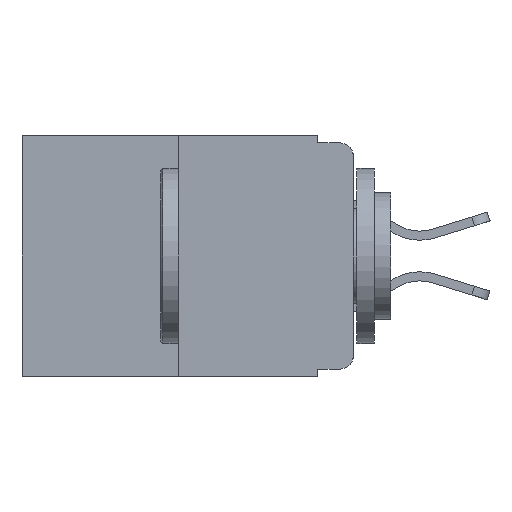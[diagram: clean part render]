
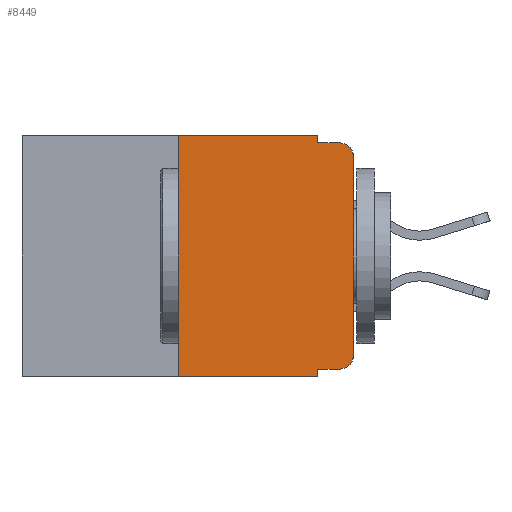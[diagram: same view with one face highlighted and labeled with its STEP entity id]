
A CAD part, left-side view. The second image highlights one B-rep face of the part: STEP entity #8449.
In plain terms, the highlighted planar face has unit normal (-1, 0, 0).
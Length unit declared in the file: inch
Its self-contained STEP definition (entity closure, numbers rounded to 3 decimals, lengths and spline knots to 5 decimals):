
#26 = CARTESIAN_POINT ( 'NONE',  ( 0., 0., -0.313 ) ) ;
#268 = ORIENTED_EDGE ( 'NONE', *, *, #11243, .T. ) ;
#380 = EDGE_CURVE ( 'NONE', #701, #8405, #5730, .T. ) ;
#486 = DIRECTION ( 'NONE',  ( 0., -1., 0. ) ) ;
#609 = CARTESIAN_POINT ( 'NONE',  ( 0., 0.051, -0.01 ) ) ;
#701 = VERTEX_POINT ( 'NONE', #7316 ) ;
#868 = LINE ( 'NONE', #9884, #1958 ) ;
#952 = CARTESIAN_POINT ( 'NONE',  ( 0., 0., -0.03 ) ) ;
#1090 = ORIENTED_EDGE ( 'NONE', *, *, #380, .F. ) ;
#1113 = DIRECTION ( 'NONE',  ( 0., 0., 1. ) ) ;
#1114 = CARTESIAN_POINT ( 'NONE',  ( 0., 0.051, 0. ) ) ;
#1180 = EDGE_CURVE ( 'NONE', #1387, #6150, #7478, .T. ) ;
#1249 = VERTEX_POINT ( 'NONE', #9430 ) ;
#1387 = VERTEX_POINT ( 'NONE', #9670 ) ;
#1479 = EDGE_LOOP ( 'NONE', ( #268, #3017, #3882, #7812, #5936, #1090, #8109, #7194, #1755, #11623 ) ) ;
#1579 = VERTEX_POINT ( 'NONE', #1114 ) ;
#1755 = ORIENTED_EDGE ( 'NONE', *, *, #5797, .T. ) ;
#1958 = VECTOR ( 'NONE', #5433, 39.37008 ) ;
#2484 = CARTESIAN_POINT ( 'NONE',  ( 0., 0.02, -0.333 ) ) ;
#2548 = LINE ( 'NONE', #6220, #4868 ) ;
#2768 = VECTOR ( 'NONE', #3510, 39.37008 ) ;
#2850 = LINE ( 'NONE', #7996, #2768 ) ;
#2852 = FACE_OUTER_BOUND ( 'NONE', #1479, .T. ) ;
#2918 = CIRCLE ( 'NONE', #11065, 0.02 ) ;
#3017 = ORIENTED_EDGE ( 'NONE', *, *, #8874, .T. ) ;
#3197 = VECTOR ( 'NONE', #4030, 39.37008 ) ;
#3454 = CARTESIAN_POINT ( 'NONE',  ( 0., 0.02, -0.313 ) ) ;
#3510 = DIRECTION ( 'NONE',  ( 0., -1., 0. ) ) ;
#3515 = EDGE_CURVE ( 'NONE', #8405, #1579, #10163, .T. ) ;
#3670 = DIRECTION ( 'NONE',  ( 0., 0., -1. ) ) ;
#3882 = ORIENTED_EDGE ( 'NONE', *, *, #10359, .F. ) ;
#3915 = DIRECTION ( 'NONE',  ( 0., 0., -1. ) ) ;
#4030 = DIRECTION ( 'NONE',  ( 0., 0., -1. ) ) ;
#4073 = EDGE_CURVE ( 'NONE', #701, #6150, #2850, .T. ) ;
#4125 = CARTESIAN_POINT ( 'NONE',  ( 0., 0.051, -0.343 ) ) ;
#4605 = CIRCLE ( 'NONE', #6100, 0.02 ) ;
#4614 = CARTESIAN_POINT ( 'NONE',  ( 0., 0.02, -0.03 ) ) ;
#4632 = AXIS2_PLACEMENT_3D ( 'NONE', #5340, #6454, #3915 ) ;
#4868 = VECTOR ( 'NONE', #5981, 39.37008 ) ;
#5340 = CARTESIAN_POINT ( 'NONE',  ( 0., 0.473, 0. ) ) ;
#5361 = VECTOR ( 'NONE', #8159, 39.37008 ) ;
#5433 = DIRECTION ( 'NONE',  ( 0., 0., -1. ) ) ;
#5444 = LINE ( 'NONE', #9062, #5361 ) ;
#5458 = PLANE ( 'NONE',  #4632 ) ;
#5513 = CARTESIAN_POINT ( 'NONE',  ( 0., 0.25, 0. ) ) ;
#5730 = LINE ( 'NONE', #9243, #7529 ) ;
#5797 = EDGE_CURVE ( 'NONE', #1387, #11275, #5444, .T. ) ;
#5936 = ORIENTED_EDGE ( 'NONE', *, *, #3515, .F. ) ;
#5981 = DIRECTION ( 'NONE',  ( 0., 0., 1. ) ) ;
#6100 = AXIS2_PLACEMENT_3D ( 'NONE', #3454, #11012, #3670 ) ;
#6150 = VERTEX_POINT ( 'NONE', #4125 ) ;
#6220 = CARTESIAN_POINT ( 'NONE',  ( 0., 0., 0. ) ) ;
#6424 = CARTESIAN_POINT ( 'NONE',  ( 0., 0.473, 0. ) ) ;
#6454 = DIRECTION ( 'NONE',  ( 1., 0., 0. ) ) ;
#7103 = DIRECTION ( 'NONE',  ( -1., 0., 0. ) ) ;
#7183 = EDGE_CURVE ( 'NONE', #11275, #10554, #4605, .T. ) ;
#7194 = ORIENTED_EDGE ( 'NONE', *, *, #1180, .F. ) ;
#7316 = CARTESIAN_POINT ( 'NONE',  ( 0., 0.25, -0.343 ) ) ;
#7478 = LINE ( 'NONE', #11265, #3197 ) ;
#7524 = EDGE_CURVE ( 'NONE', #1579, #1249, #868, .T. ) ;
#7529 = VECTOR ( 'NONE', #1113, 39.37008 ) ;
#7812 = ORIENTED_EDGE ( 'NONE', *, *, #7524, .F. ) ;
#7939 = VERTEX_POINT ( 'NONE', #8973 ) ;
#7996 = CARTESIAN_POINT ( 'NONE',  ( 0., 0.473, -0.343 ) ) ;
#8109 = ORIENTED_EDGE ( 'NONE', *, *, #4073, .T. ) ;
#8159 = DIRECTION ( 'NONE',  ( 0., -1., 0. ) ) ;
#8214 = VECTOR ( 'NONE', #9209, 39.37008 ) ;
#8405 = VERTEX_POINT ( 'NONE', #5513 ) ;
#8423 = VERTEX_POINT ( 'NONE', #952 ) ;
#8449 = ADVANCED_FACE ( 'NONE', ( #2852 ), #5458, .F. ) ;
#8874 = EDGE_CURVE ( 'NONE', #8423, #7939, #2918, .T. ) ;
#8973 = CARTESIAN_POINT ( 'NONE',  ( 0., 0.02, -0.01 ) ) ;
#9013 = VECTOR ( 'NONE', #486, 39.37008 ) ;
#9062 = CARTESIAN_POINT ( 'NONE',  ( 0., 0.051, -0.333 ) ) ;
#9209 = DIRECTION ( 'NONE',  ( 0., -1., 0. ) ) ;
#9243 = CARTESIAN_POINT ( 'NONE',  ( 0., 0.25, 0. ) ) ;
#9430 = CARTESIAN_POINT ( 'NONE',  ( 0., 0.051, -0.01 ) ) ;
#9670 = CARTESIAN_POINT ( 'NONE',  ( 0., 0.051, -0.333 ) ) ;
#9702 = LINE ( 'NONE', #609, #9013 ) ;
#9838 = DIRECTION ( 'NONE',  ( 0., 0., -1. ) ) ;
#9884 = CARTESIAN_POINT ( 'NONE',  ( 0., 0.051, 0. ) ) ;
#10163 = LINE ( 'NONE', #6424, #8214 ) ;
#10359 = EDGE_CURVE ( 'NONE', #1249, #7939, #9702, .T. ) ;
#10554 = VERTEX_POINT ( 'NONE', #26 ) ;
#11012 = DIRECTION ( 'NONE',  ( -1., 0., 0. ) ) ;
#11065 = AXIS2_PLACEMENT_3D ( 'NONE', #4614, #7103, #9838 ) ;
#11243 = EDGE_CURVE ( 'NONE', #10554, #8423, #2548, .T. ) ;
#11265 = CARTESIAN_POINT ( 'NONE',  ( 0., 0.051, 0. ) ) ;
#11275 = VERTEX_POINT ( 'NONE', #2484 ) ;
#11623 = ORIENTED_EDGE ( 'NONE', *, *, #7183, .T. ) ;
